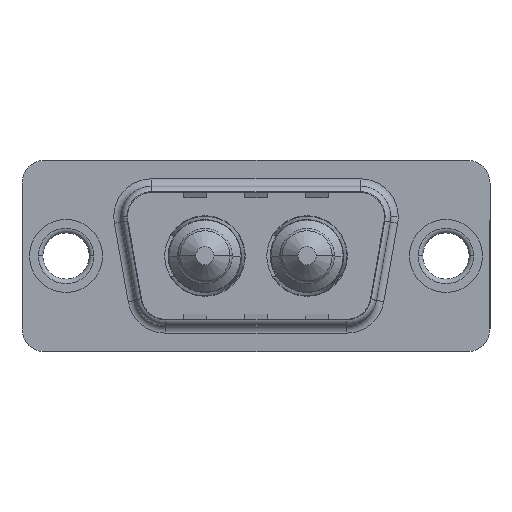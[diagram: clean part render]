
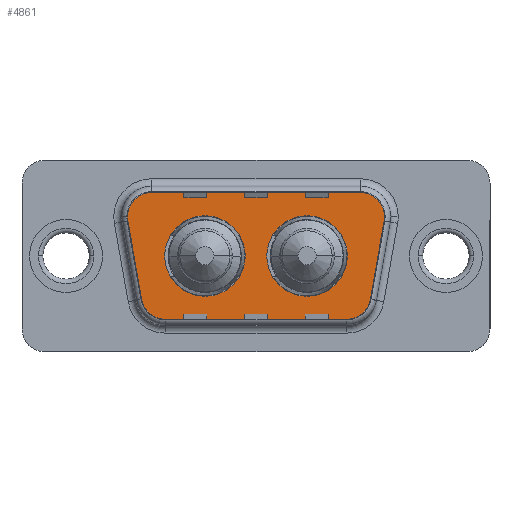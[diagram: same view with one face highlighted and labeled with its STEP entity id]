
A CAD part, top view. The second image highlights one B-rep face of the part: STEP entity #4861.
In plain terms, the highlighted planar face has unit normal (0, 0, 1).
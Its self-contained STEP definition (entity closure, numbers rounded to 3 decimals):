
#85 = EDGE_LOOP ( 'NONE', ( #7638, #2435 ) ) ;
#156 = CARTESIAN_POINT ( 'NONE',  ( 3.466, 2.553, 0. ) ) ;
#261 = CARTESIAN_POINT ( 'NONE',  ( 13.21, 0., 0. ) ) ;
#392 = VERTEX_POINT ( 'NONE', #5771 ) ;
#460 = LINE ( 'NONE', #156, #4172 ) ;
#543 = DIRECTION ( 'NONE',  ( 0., 0., 1. ) ) ;
#773 = DIRECTION ( 'NONE',  ( 1., 0., 0. ) ) ;
#877 = ORIENTED_EDGE ( 'NONE', *, *, #1253, .F. ) ;
#1064 = CARTESIAN_POINT ( 'NONE',  ( 6.49, 0., 0. ) ) ;
#1124 = EDGE_CURVE ( 'NONE', #392, #2248, #8875, .T. ) ;
#1185 = CIRCLE ( 'NONE', #4786, 2. ) ;
#1243 = ORIENTED_EDGE ( 'NONE', *, *, #1997, .T. ) ;
#1253 = EDGE_CURVE ( 'NONE', #8718, #1633, #4202, .T. ) ;
#1259 = CIRCLE ( 'NONE', #2171, 2. ) ;
#1310 = DIRECTION ( 'NONE',  ( 1., 0., 0. ) ) ;
#1350 = CARTESIAN_POINT ( 'NONE',  ( 9.14, 0., 0. ) ) ;
#1501 = DIRECTION ( 'NONE',  ( -1., 0., 0. ) ) ;
#1633 = VERTEX_POINT ( 'NONE', #261 ) ;
#1867 = VECTOR ( 'NONE', #1501, 1000. ) ;
#1997 = EDGE_CURVE ( 'NONE', #2074, #5197, #5809, .T. ) ;
#2074 = VERTEX_POINT ( 'NONE', #4200 ) ;
#2088 = ORIENTED_EDGE ( 'NONE', *, *, #2207, .T. ) ;
#2171 = AXIS2_PLACEMENT_3D ( 'NONE', #7567, #5755, #1310 ) ;
#2188 = CARTESIAN_POINT ( 'NONE',  ( 5.436, 4.9, 0. ) ) ;
#2207 = EDGE_CURVE ( 'NONE', #3018, #5575, #460, .T. ) ;
#2248 = VERTEX_POINT ( 'NONE', #6659 ) ;
#2331 = EDGE_LOOP ( 'NONE', ( #877, #4592 ) ) ;
#2342 = ORIENTED_EDGE ( 'NONE', *, *, #6304, .T. ) ;
#2352 = DIRECTION ( 'NONE',  ( 1., 0., 0. ) ) ;
#2435 = ORIENTED_EDGE ( 'NONE', *, *, #5559, .F. ) ;
#2473 = CIRCLE ( 'NONE', #9666, 2.65 ) ;
#2509 = ORIENTED_EDGE ( 'NONE', *, *, #3594, .T. ) ;
#2529 = ORIENTED_EDGE ( 'NONE', *, *, #8277, .T. ) ;
#2600 = AXIS2_PLACEMENT_3D ( 'NONE', #8904, #4433, #9642 ) ;
#2800 = AXIS2_PLACEMENT_3D ( 'NONE', #9675, #9535, #9467 ) ;
#2867 = EDGE_CURVE ( 'NONE', #5197, #3018, #1259, .T. ) ;
#2928 = CARTESIAN_POINT ( 'NONE',  ( 19.564, 2.9, 0. ) ) ;
#2950 = CARTESIAN_POINT ( 'NONE',  ( 18.541, -2.9, 0. ) ) ;
#3018 = VERTEX_POINT ( 'NONE', #9016 ) ;
#3083 = VERTEX_POINT ( 'NONE', #9613 ) ;
#3098 = DIRECTION ( 'NONE',  ( 0.174, 0.985, 0. ) ) ;
#3182 = DIRECTION ( 'NONE',  ( 1., 0., 0. ) ) ;
#3222 = EDGE_CURVE ( 'NONE', #5731, #9326, #7620, .T. ) ;
#3279 = CARTESIAN_POINT ( 'NONE',  ( 9.14, 0., 0. ) ) ;
#3410 = VERTEX_POINT ( 'NONE', #9361 ) ;
#3415 = DIRECTION ( 'NONE',  ( 0., 0., 1. ) ) ;
#3569 = DIRECTION ( 'NONE',  ( -1., 0., 0. ) ) ;
#3594 = EDGE_CURVE ( 'NONE', #3410, #392, #8531, .T. ) ;
#3628 = DIRECTION ( 'NONE',  ( 0., 0., 1. ) ) ;
#3710 = AXIS2_PLACEMENT_3D ( 'NONE', #2950, #543, #3182 ) ;
#3840 = EDGE_CURVE ( 'NONE', #1633, #8718, #2473, .T. ) ;
#4172 = VECTOR ( 'NONE', #6796, 1000. ) ;
#4191 = CARTESIAN_POINT ( 'NONE',  ( 18.51, 0., 0. ) ) ;
#4193 = FACE_BOUND ( 'NONE', #85, .T. ) ;
#4200 = CARTESIAN_POINT ( 'NONE',  ( 19.564, 4.9, 0. ) ) ;
#4202 = CIRCLE ( 'NONE', #2800, 2.65 ) ;
#4300 = EDGE_CURVE ( 'NONE', #9357, #3410, #1185, .T. ) ;
#4432 = FACE_BOUND ( 'NONE', #2331, .T. ) ;
#4433 = DIRECTION ( 'NONE',  ( 0., 0., 1. ) ) ;
#4560 = EDGE_CURVE ( 'NONE', #5575, #3083, #5478, .T. ) ;
#4592 = ORIENTED_EDGE ( 'NONE', *, *, #3840, .F. ) ;
#4786 = AXIS2_PLACEMENT_3D ( 'NONE', #5569, #5555, #773 ) ;
#4861 = ADVANCED_FACE ( 'NONE', ( #4432, #4193, #7916 ), #5433, .T. ) ;
#5036 = AXIS2_PLACEMENT_3D ( 'NONE', #1350, #6635, #2352 ) ;
#5197 = VERTEX_POINT ( 'NONE', #2188 ) ;
#5321 = ORIENTED_EDGE ( 'NONE', *, *, #2867, .T. ) ;
#5349 = LINE ( 'NONE', #8995, #9089 ) ;
#5416 = CIRCLE ( 'NONE', #2600, 2. ) ;
#5433 = PLANE ( 'NONE',  #3710 ) ;
#5478 = CIRCLE ( 'NONE', #7584, 2. ) ;
#5555 = DIRECTION ( 'NONE',  ( 0., 0., 1. ) ) ;
#5559 = EDGE_CURVE ( 'NONE', #9326, #5731, #9455, .T. ) ;
#5569 = CARTESIAN_POINT ( 'NONE',  ( 18.541, -2.9, 0. ) ) ;
#5575 = VERTEX_POINT ( 'NONE', #6448 ) ;
#5731 = VERTEX_POINT ( 'NONE', #9223 ) ;
#5755 = DIRECTION ( 'NONE',  ( 0., 0., 1. ) ) ;
#5762 = ORIENTED_EDGE ( 'NONE', *, *, #4300, .T. ) ;
#5771 = CARTESIAN_POINT ( 'NONE',  ( 21.534, 2.553, 0. ) ) ;
#5809 = LINE ( 'NONE', #9662, #1867 ) ;
#5869 = DIRECTION ( 'NONE',  ( -1., 0., 0. ) ) ;
#6304 = EDGE_CURVE ( 'NONE', #3083, #9357, #5349, .T. ) ;
#6306 = CARTESIAN_POINT ( 'NONE',  ( 18.541, -4.9, 0. ) ) ;
#6448 = CARTESIAN_POINT ( 'NONE',  ( 4.489, -3.247, 0. ) ) ;
#6635 = DIRECTION ( 'NONE',  ( 0., 0., 1. ) ) ;
#6659 = CARTESIAN_POINT ( 'NONE',  ( 21.564, 2.9, 0. ) ) ;
#6796 = DIRECTION ( 'NONE',  ( 0.174, -0.985, 0. ) ) ;
#6908 = ORIENTED_EDGE ( 'NONE', *, *, #1124, .T. ) ;
#7380 = CARTESIAN_POINT ( 'NONE',  ( 6.459, -2.9, 0. ) ) ;
#7559 = CARTESIAN_POINT ( 'NONE',  ( 21.534, 2.553, 0. ) ) ;
#7567 = CARTESIAN_POINT ( 'NONE',  ( 5.436, 2.9, 0. ) ) ;
#7584 = AXIS2_PLACEMENT_3D ( 'NONE', #7380, #7802, #3569 ) ;
#7620 = CIRCLE ( 'NONE', #5036, 2.65 ) ;
#7638 = ORIENTED_EDGE ( 'NONE', *, *, #3222, .F. ) ;
#7802 = DIRECTION ( 'NONE',  ( 0., 0., 1. ) ) ;
#7900 = CARTESIAN_POINT ( 'NONE',  ( 15.86, 0., 0. ) ) ;
#7916 = FACE_OUTER_BOUND ( 'NONE', #8700, .T. ) ;
#7944 = AXIS2_PLACEMENT_3D ( 'NONE', #2928, #3628, #5869 ) ;
#8058 = VECTOR ( 'NONE', #3098, 1000. ) ;
#8277 = EDGE_CURVE ( 'NONE', #2248, #2074, #5416, .T. ) ;
#8494 = DIRECTION ( 'NONE',  ( 1., 0., 0. ) ) ;
#8531 = LINE ( 'NONE', #7559, #8058 ) ;
#8700 = EDGE_LOOP ( 'NONE', ( #5762, #2509, #6908, #2529, #1243, #5321, #2088, #9561, #2342 ) ) ;
#8718 = VERTEX_POINT ( 'NONE', #4191 ) ;
#8875 = CIRCLE ( 'NONE', #7944, 2. ) ;
#8904 = CARTESIAN_POINT ( 'NONE',  ( 19.564, 2.9, 0. ) ) ;
#8995 = CARTESIAN_POINT ( 'NONE',  ( 6.459, -4.9, 0. ) ) ;
#9016 = CARTESIAN_POINT ( 'NONE',  ( 3.466, 2.553, 0. ) ) ;
#9054 = DIRECTION ( 'NONE',  ( 1., 0., 0. ) ) ;
#9089 = VECTOR ( 'NONE', #8494, 1000. ) ;
#9223 = CARTESIAN_POINT ( 'NONE',  ( 11.79, 0., 0. ) ) ;
#9326 = VERTEX_POINT ( 'NONE', #1064 ) ;
#9357 = VERTEX_POINT ( 'NONE', #6306 ) ;
#9361 = CARTESIAN_POINT ( 'NONE',  ( 20.511, -3.247, 0. ) ) ;
#9365 = AXIS2_PLACEMENT_3D ( 'NONE', #3279, #9418, #9406 ) ;
#9406 = DIRECTION ( 'NONE',  ( 1., 0., 0. ) ) ;
#9418 = DIRECTION ( 'NONE',  ( 0., 0., 1. ) ) ;
#9455 = CIRCLE ( 'NONE', #9365, 2.65 ) ;
#9467 = DIRECTION ( 'NONE',  ( 1., 0., 0. ) ) ;
#9535 = DIRECTION ( 'NONE',  ( 0., 0., 1. ) ) ;
#9561 = ORIENTED_EDGE ( 'NONE', *, *, #4560, .T. ) ;
#9613 = CARTESIAN_POINT ( 'NONE',  ( 6.459, -4.9, 0. ) ) ;
#9642 = DIRECTION ( 'NONE',  ( -1., 0., 0. ) ) ;
#9662 = CARTESIAN_POINT ( 'NONE',  ( 5.436, 4.9, 0. ) ) ;
#9666 = AXIS2_PLACEMENT_3D ( 'NONE', #7900, #3415, #9054 ) ;
#9675 = CARTESIAN_POINT ( 'NONE',  ( 15.86, 0., 0. ) ) ;
